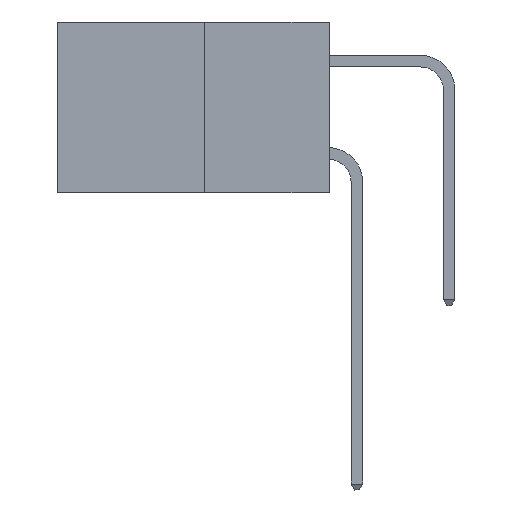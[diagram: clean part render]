
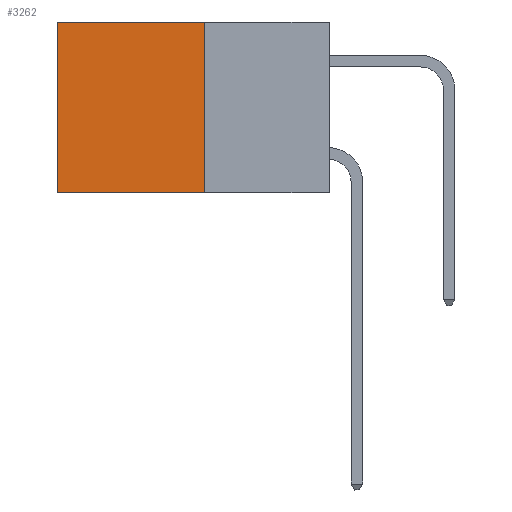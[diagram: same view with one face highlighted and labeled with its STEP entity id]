
A CAD part, left-side view. The second image highlights one B-rep face of the part: STEP entity #3262.
In plain terms, the highlighted planar face has unit normal (-1, 0, 0).
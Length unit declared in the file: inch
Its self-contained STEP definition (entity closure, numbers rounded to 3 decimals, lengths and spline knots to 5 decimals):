
#572 = CARTESIAN_POINT ( 'NONE',  ( 0.277, 0.27, 0. ) ) ;
#1075 = ORIENTED_EDGE ( 'NONE', *, *, #7455, .F. ) ;
#1128 = CARTESIAN_POINT ( 'NONE',  ( 0.277, 0.27, -0.37 ) ) ;
#1491 = DIRECTION ( 'NONE',  ( 0., 0., -1. ) ) ;
#1548 = CARTESIAN_POINT ( 'NONE',  ( 0.277, 0.27, -0.37 ) ) ;
#2081 = EDGE_CURVE ( 'NONE', #3573, #25192, #17048, .T. ) ;
#2416 = ORIENTED_EDGE ( 'NONE', *, *, #26353, .F. ) ;
#2429 = VECTOR ( 'NONE', #1491, 39.37008 ) ;
#2783 = VECTOR ( 'NONE', #7086, 39.37008 ) ;
#3262 = ADVANCED_FACE ( 'NONE', ( #16627 ), #12385, .F. ) ;
#3384 = DIRECTION ( 'NONE',  ( 0., 0., -1. ) ) ;
#3573 = VERTEX_POINT ( 'NONE', #17810 ) ;
#3878 = VECTOR ( 'NONE', #16038, 39.37008 ) ;
#4798 = CARTESIAN_POINT ( 'NONE',  ( 0.277, 0.27, -0.37 ) ) ;
#5367 = CARTESIAN_POINT ( 'NONE',  ( 0.277, 0.59, 0. ) ) ;
#7086 = DIRECTION ( 'NONE',  ( 0., 0., -1. ) ) ;
#7455 = EDGE_CURVE ( 'NONE', #17498, #28321, #21033, .T. ) ;
#8449 = LINE ( 'NONE', #28191, #2429 ) ;
#11094 = VECTOR ( 'NONE', #28533, 39.37008 ) ;
#11909 = ORIENTED_EDGE ( 'NONE', *, *, #16779, .T. ) ;
#12385 = PLANE ( 'NONE',  #14171 ) ;
#13760 = CARTESIAN_POINT ( 'NONE',  ( 0.277, 0.27, -0.37 ) ) ;
#14171 = AXIS2_PLACEMENT_3D ( 'NONE', #1128, #16863, #3384 ) ;
#16038 = DIRECTION ( 'NONE',  ( 0., 1., 0. ) ) ;
#16627 = FACE_OUTER_BOUND ( 'NONE', #25808, .T. ) ;
#16779 = EDGE_CURVE ( 'NONE', #25192, #28321, #8449, .T. ) ;
#16863 = DIRECTION ( 'NONE',  ( 1., 0., 0. ) ) ;
#17048 = LINE ( 'NONE', #572, #11094 ) ;
#17498 = VERTEX_POINT ( 'NONE', #1548 ) ;
#17810 = CARTESIAN_POINT ( 'NONE',  ( 0.277, 0.27, 0. ) ) ;
#20653 = LINE ( 'NONE', #4798, #2783 ) ;
#21033 = LINE ( 'NONE', #13760, #3878 ) ;
#21067 = ORIENTED_EDGE ( 'NONE', *, *, #2081, .T. ) ;
#25192 = VERTEX_POINT ( 'NONE', #5367 ) ;
#25808 = EDGE_LOOP ( 'NONE', ( #11909, #1075, #2416, #21067 ) ) ;
#26353 = EDGE_CURVE ( 'NONE', #3573, #17498, #20653, .T. ) ;
#27300 = CARTESIAN_POINT ( 'NONE',  ( 0.277, 0.59, -0.37 ) ) ;
#28191 = CARTESIAN_POINT ( 'NONE',  ( 0.277, 0.59, -0.37 ) ) ;
#28321 = VERTEX_POINT ( 'NONE', #27300 ) ;
#28533 = DIRECTION ( 'NONE',  ( 0., 1., 0. ) ) ;
